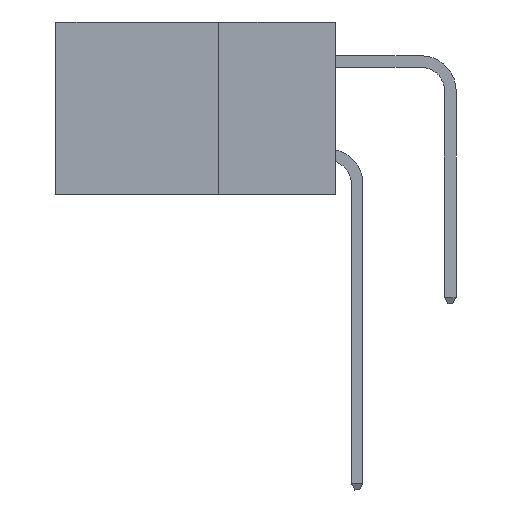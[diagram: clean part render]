
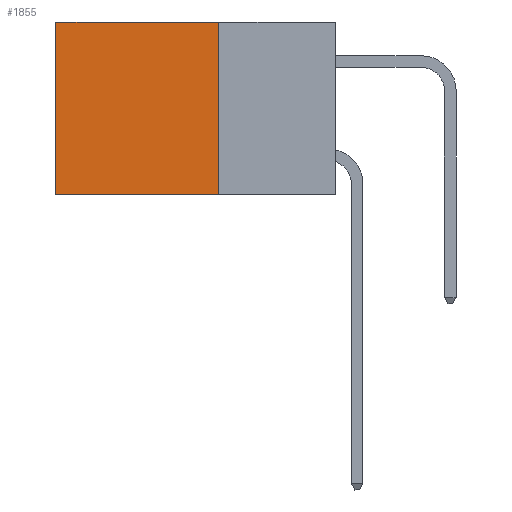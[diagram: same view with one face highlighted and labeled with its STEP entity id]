
A CAD part, left-side view. The second image highlights one B-rep face of the part: STEP entity #1855.
In plain terms, the highlighted planar face has unit normal (-1, 0, 0).
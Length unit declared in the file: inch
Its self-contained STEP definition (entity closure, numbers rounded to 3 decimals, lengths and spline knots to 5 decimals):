
#1579 = PLANE ( 'NONE',  #18824 ) ;
#1622 = LINE ( 'NONE', #12684, #13582 ) ;
#1855 = ADVANCED_FACE ( 'NONE', ( #21479 ), #1579, .F. ) ;
#3348 = LINE ( 'NONE', #17285, #20966 ) ;
#3421 = VERTEX_POINT ( 'NONE', #20006 ) ;
#3980 = VECTOR ( 'NONE', #21070, 39.37008 ) ;
#4003 = CARTESIAN_POINT ( 'NONE',  ( 0.2875, 0.6, 0. ) ) ;
#4138 = ORIENTED_EDGE ( 'NONE', *, *, #5875, .T. ) ;
#4440 = VECTOR ( 'NONE', #14189, 39.37008 ) ;
#5558 = EDGE_CURVE ( 'NONE', #20745, #11775, #1622, .T. ) ;
#5875 = EDGE_CURVE ( 'NONE', #3421, #6400, #22414, .T. ) ;
#6400 = VERTEX_POINT ( 'NONE', #19447 ) ;
#7287 = ORIENTED_EDGE ( 'NONE', *, *, #19346, .T. ) ;
#7313 = CARTESIAN_POINT ( 'NONE',  ( 0.2875, 0.25, 0. ) ) ;
#7377 = DIRECTION ( 'NONE',  ( 1., 0., 0. ) ) ;
#9293 = LINE ( 'NONE', #25197, #3980 ) ;
#11775 = VERTEX_POINT ( 'NONE', #19070 ) ;
#12684 = CARTESIAN_POINT ( 'NONE',  ( 0.2875, 0.25, 0. ) ) ;
#13027 = DIRECTION ( 'NONE',  ( 0., 0., -1. ) ) ;
#13359 = CARTESIAN_POINT ( 'NONE',  ( 0.2875, 0.25, 0. ) ) ;
#13540 = DIRECTION ( 'NONE',  ( 0., 0., -1. ) ) ;
#13582 = VECTOR ( 'NONE', #13027, 39.37008 ) ;
#14189 = DIRECTION ( 'NONE',  ( 0., 0., -1. ) ) ;
#14921 = EDGE_CURVE ( 'NONE', #11775, #6400, #3348, .T. ) ;
#17285 = CARTESIAN_POINT ( 'NONE',  ( 0.2875, 0.25, -0.37 ) ) ;
#18824 = AXIS2_PLACEMENT_3D ( 'NONE', #13359, #7377, #13540 ) ;
#19070 = CARTESIAN_POINT ( 'NONE',  ( 0.2875, 0.25, -0.37 ) ) ;
#19346 = EDGE_CURVE ( 'NONE', #20745, #3421, #9293, .T. ) ;
#19447 = CARTESIAN_POINT ( 'NONE',  ( 0.2875, 0.6, -0.37 ) ) ;
#20006 = CARTESIAN_POINT ( 'NONE',  ( 0.2875, 0.6, 0. ) ) ;
#20745 = VERTEX_POINT ( 'NONE', #7313 ) ;
#20966 = VECTOR ( 'NONE', #23440, 39.37008 ) ;
#21070 = DIRECTION ( 'NONE',  ( 0., 1., 0. ) ) ;
#21479 = FACE_OUTER_BOUND ( 'NONE', #22927, .T. ) ;
#22414 = LINE ( 'NONE', #4003, #4440 ) ;
#22927 = EDGE_LOOP ( 'NONE', ( #4138, #24867, #24119, #7287 ) ) ;
#23440 = DIRECTION ( 'NONE',  ( 0., 1., 0. ) ) ;
#24119 = ORIENTED_EDGE ( 'NONE', *, *, #5558, .F. ) ;
#24867 = ORIENTED_EDGE ( 'NONE', *, *, #14921, .F. ) ;
#25197 = CARTESIAN_POINT ( 'NONE',  ( 0.2875, 0.25, 0. ) ) ;
